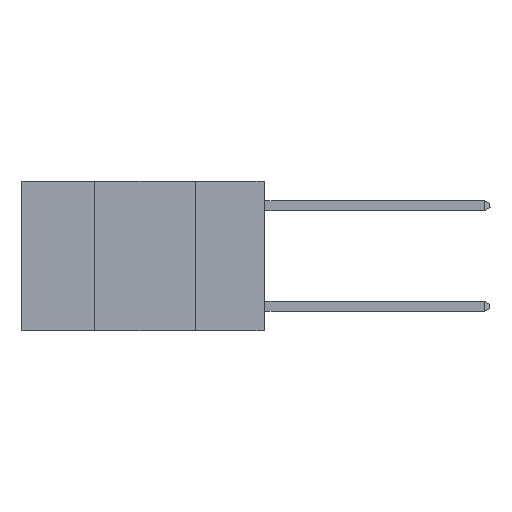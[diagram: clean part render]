
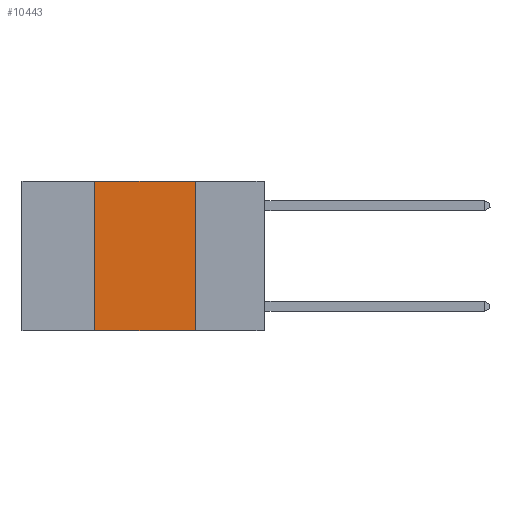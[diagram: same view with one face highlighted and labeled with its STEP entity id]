
A CAD part, left-side view. The second image highlights one B-rep face of the part: STEP entity #10443.
In plain terms, the highlighted planar face has unit normal (-1, 0, 0).
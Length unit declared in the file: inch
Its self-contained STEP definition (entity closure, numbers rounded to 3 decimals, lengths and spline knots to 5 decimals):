
#613 = CARTESIAN_POINT ( 'NONE',  ( 0., 0.17, 0. ) ) ;
#897 = DIRECTION ( 'NONE',  ( 0., -1., 0. ) ) ;
#968 = VECTOR ( 'NONE', #12584, 39.37008 ) ;
#1405 = VERTEX_POINT ( 'NONE', #19253 ) ;
#2928 = VECTOR ( 'NONE', #7613, 39.37008 ) ;
#3203 = EDGE_CURVE ( 'NONE', #8365, #18203, #18042, .T. ) ;
#3426 = CARTESIAN_POINT ( 'NONE',  ( 0., 0.17, -0.37 ) ) ;
#4621 = DIRECTION ( 'NONE',  ( 1., 0., 0. ) ) ;
#5107 = AXIS2_PLACEMENT_3D ( 'NONE', #10558, #4621, #15048 ) ;
#5721 = CARTESIAN_POINT ( 'NONE',  ( 0., 0.42, 0. ) ) ;
#6084 = CARTESIAN_POINT ( 'NONE',  ( 0., 0.6, -0.37 ) ) ;
#7384 = LINE ( 'NONE', #6084, #2928 ) ;
#7613 = DIRECTION ( 'NONE',  ( 0., -1., 0. ) ) ;
#7955 = ORIENTED_EDGE ( 'NONE', *, *, #3203, .F. ) ;
#8002 = ORIENTED_EDGE ( 'NONE', *, *, #11726, .F. ) ;
#8090 = EDGE_CURVE ( 'NONE', #18203, #14001, #9377, .T. ) ;
#8276 = ORIENTED_EDGE ( 'NONE', *, *, #8090, .F. ) ;
#8365 = VERTEX_POINT ( 'NONE', #5721 ) ;
#8638 = FACE_OUTER_BOUND ( 'NONE', #10941, .T. ) ;
#9030 = PLANE ( 'NONE',  #5107 ) ;
#9212 = DIRECTION ( 'NONE',  ( 0., 0., 1. ) ) ;
#9377 = LINE ( 'NONE', #613, #968 ) ;
#10443 = ADVANCED_FACE ( 'NONE', ( #8638 ), #9030, .F. ) ;
#10558 = CARTESIAN_POINT ( 'NONE',  ( 0., 0.6, 0. ) ) ;
#10941 = EDGE_LOOP ( 'NONE', ( #8276, #7955, #8002, #17949 ) ) ;
#11383 = CARTESIAN_POINT ( 'NONE',  ( 0., 0.6, 0. ) ) ;
#11726 = EDGE_CURVE ( 'NONE', #1405, #8365, #18335, .T. ) ;
#12584 = DIRECTION ( 'NONE',  ( 0., 0., -1. ) ) ;
#13706 = EDGE_CURVE ( 'NONE', #1405, #14001, #7384, .T. ) ;
#13948 = VECTOR ( 'NONE', #9212, 39.37008 ) ;
#14001 = VERTEX_POINT ( 'NONE', #3426 ) ;
#14123 = VECTOR ( 'NONE', #897, 39.37008 ) ;
#15048 = DIRECTION ( 'NONE',  ( 0., 0., -1. ) ) ;
#16643 = CARTESIAN_POINT ( 'NONE',  ( 0., 0.42, 0. ) ) ;
#17949 = ORIENTED_EDGE ( 'NONE', *, *, #13706, .T. ) ;
#18042 = LINE ( 'NONE', #11383, #14123 ) ;
#18137 = CARTESIAN_POINT ( 'NONE',  ( 0., 0.17, 0. ) ) ;
#18203 = VERTEX_POINT ( 'NONE', #18137 ) ;
#18335 = LINE ( 'NONE', #16643, #13948 ) ;
#19253 = CARTESIAN_POINT ( 'NONE',  ( 0., 0.42, -0.37 ) ) ;
